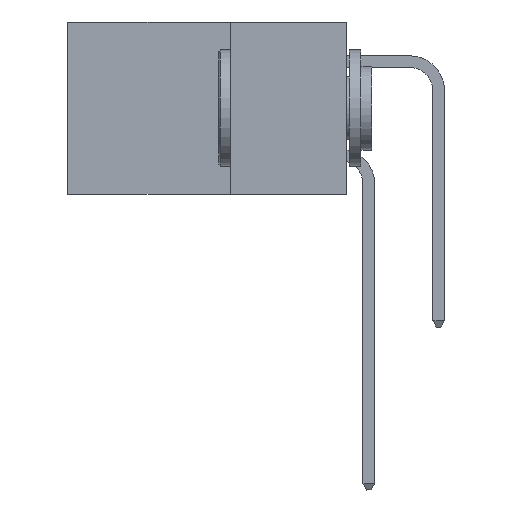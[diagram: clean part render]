
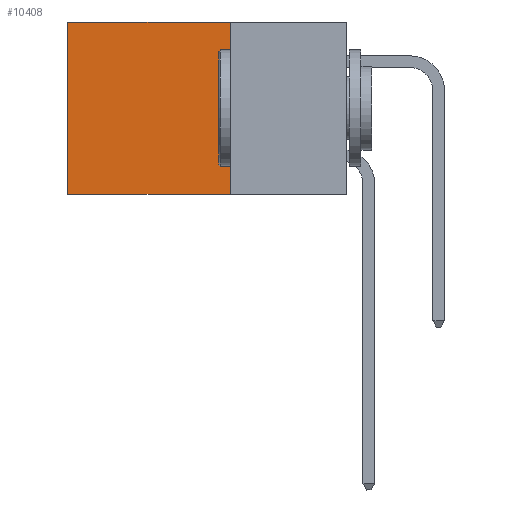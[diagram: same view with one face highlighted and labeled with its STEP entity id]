
A CAD part, left-side view. The second image highlights one B-rep face of the part: STEP entity #10408.
In plain terms, the highlighted planar face has unit normal (-1, 0, 0).
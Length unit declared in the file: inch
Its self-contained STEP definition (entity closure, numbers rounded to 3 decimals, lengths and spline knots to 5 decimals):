
#394 = VERTEX_POINT ( 'NONE', #23575 ) ;
#1169 = DIRECTION ( 'NONE',  ( 0., 0., -1. ) ) ;
#1280 = EDGE_CURVE ( 'NONE', #2734, #21762, #17142, .T. ) ;
#2734 = VERTEX_POINT ( 'NONE', #17572 ) ;
#3829 = ORIENTED_EDGE ( 'NONE', *, *, #23651, .F. ) ;
#5712 = FACE_OUTER_BOUND ( 'NONE', #17201, .T. ) ;
#6480 = CARTESIAN_POINT ( 'NONE',  ( 0.2875, 0.6, -0.37 ) ) ;
#7327 = PLANE ( 'NONE',  #22767 ) ;
#7486 = CARTESIAN_POINT ( 'NONE',  ( 0.2875, 0.25, 0. ) ) ;
#7894 = LINE ( 'NONE', #15391, #22624 ) ;
#7921 = CARTESIAN_POINT ( 'NONE',  ( 0.2875, 0.25, -0.37 ) ) ;
#8035 = LINE ( 'NONE', #8753, #16439 ) ;
#8753 = CARTESIAN_POINT ( 'NONE',  ( 0.2875, 0.6, 0. ) ) ;
#8940 = ORIENTED_EDGE ( 'NONE', *, *, #1280, .F. ) ;
#9132 = CARTESIAN_POINT ( 'NONE',  ( 0.2875, 0.25, 0. ) ) ;
#9476 = DIRECTION ( 'NONE',  ( 0., 0., -1. ) ) ;
#9592 = EDGE_CURVE ( 'NONE', #2734, #394, #7894, .T. ) ;
#9957 = VECTOR ( 'NONE', #9476, 39.37008 ) ;
#10408 = ADVANCED_FACE ( 'NONE', ( #5712 ), #7327, .F. ) ;
#10519 = DIRECTION ( 'NONE',  ( 0., 1., 0. ) ) ;
#13260 = ORIENTED_EDGE ( 'NONE', *, *, #22955, .T. ) ;
#15391 = CARTESIAN_POINT ( 'NONE',  ( 0.2875, 0.25, 0. ) ) ;
#16439 = VECTOR ( 'NONE', #1169, 39.37008 ) ;
#16789 = VERTEX_POINT ( 'NONE', #6480 ) ;
#17142 = LINE ( 'NONE', #9132, #9957 ) ;
#17201 = EDGE_LOOP ( 'NONE', ( #13260, #3829, #8940, #24771 ) ) ;
#17572 = CARTESIAN_POINT ( 'NONE',  ( 0.2875, 0.25, 0. ) ) ;
#18599 = CARTESIAN_POINT ( 'NONE',  ( 0.2875, 0.25, -0.37 ) ) ;
#19195 = DIRECTION ( 'NONE',  ( 0., 1., 0. ) ) ;
#20625 = LINE ( 'NONE', #18599, #21519 ) ;
#21519 = VECTOR ( 'NONE', #10519, 39.37008 ) ;
#21762 = VERTEX_POINT ( 'NONE', #7921 ) ;
#22609 = DIRECTION ( 'NONE',  ( 0., 0., -1. ) ) ;
#22624 = VECTOR ( 'NONE', #19195, 39.37008 ) ;
#22767 = AXIS2_PLACEMENT_3D ( 'NONE', #7486, #24767, #22609 ) ;
#22955 = EDGE_CURVE ( 'NONE', #394, #16789, #8035, .T. ) ;
#23575 = CARTESIAN_POINT ( 'NONE',  ( 0.2875, 0.6, 0. ) ) ;
#23651 = EDGE_CURVE ( 'NONE', #21762, #16789, #20625, .T. ) ;
#24767 = DIRECTION ( 'NONE',  ( 1., 0., 0. ) ) ;
#24771 = ORIENTED_EDGE ( 'NONE', *, *, #9592, .T. ) ;
